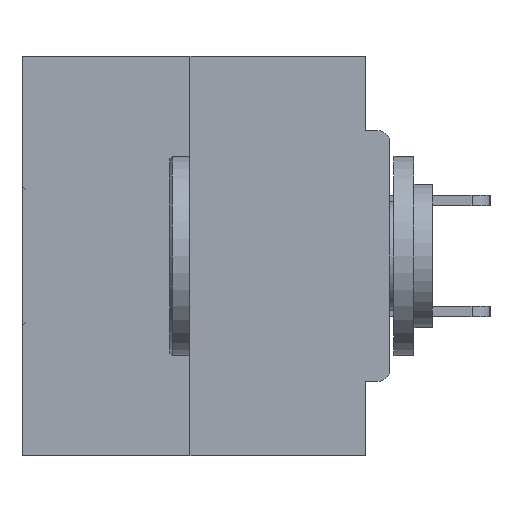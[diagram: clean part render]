
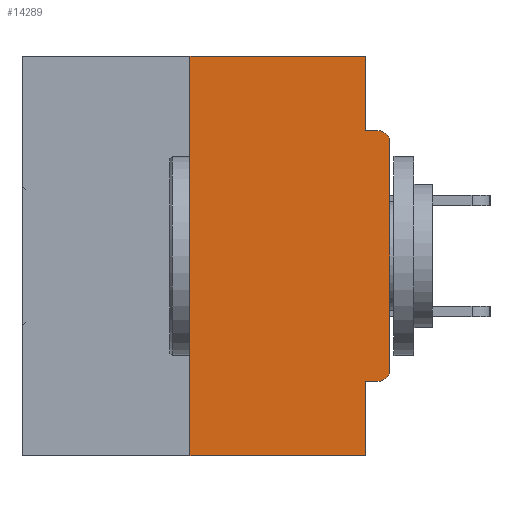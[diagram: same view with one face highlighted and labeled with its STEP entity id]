
A CAD part, left-side view. The second image highlights one B-rep face of the part: STEP entity #14289.
In plain terms, the highlighted planar face has unit normal (-1, 0, 0).
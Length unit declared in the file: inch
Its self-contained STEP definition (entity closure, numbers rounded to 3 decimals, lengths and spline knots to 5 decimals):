
#1080 = EDGE_CURVE ( 'NONE', #7391, #29625, #39101, .T. ) ;
#1329 = ORIENTED_EDGE ( 'NONE', *, *, #24493, .F. ) ;
#1868 = PLANE ( 'NONE',  #25152 ) ;
#2980 = VERTEX_POINT ( 'NONE', #11362 ) ;
#3025 = CARTESIAN_POINT ( 'NONE',  ( 0., 0.031, -0.5 ) ) ;
#3159 = CARTESIAN_POINT ( 'NONE',  ( 0., 0.015, -0.3915 ) ) ;
#3633 = EDGE_CURVE ( 'NONE', #15242, #29625, #30633, .T. ) ;
#3781 = EDGE_LOOP ( 'NONE', ( #1329, #34280, #20419, #6458, #30630, #20638, #4569, #37839, #4929, #18616 ) ) ;
#3794 = DIRECTION ( 'NONE',  ( 0., 0., -1. ) ) ;
#4330 = CARTESIAN_POINT ( 'NONE',  ( 0., 0., -0.1085 ) ) ;
#4569 = ORIENTED_EDGE ( 'NONE', *, *, #7837, .T. ) ;
#4770 = DIRECTION ( 'NONE',  ( 1., 0., 0. ) ) ;
#4929 = ORIENTED_EDGE ( 'NONE', *, *, #3633, .F. ) ;
#6458 = ORIENTED_EDGE ( 'NONE', *, *, #23088, .F. ) ;
#7391 = VERTEX_POINT ( 'NONE', #4330 ) ;
#7837 = EDGE_CURVE ( 'NONE', #17919, #7391, #25244, .T. ) ;
#8629 = LINE ( 'NONE', #20270, #10664 ) ;
#10664 = VECTOR ( 'NONE', #23188, 39.37008 ) ;
#10782 = CIRCLE ( 'NONE', #37553, 0.015 ) ;
#10955 = LINE ( 'NONE', #12834, #26357 ) ;
#11361 = DIRECTION ( 'NONE',  ( 0., 0., -1. ) ) ;
#11362 = CARTESIAN_POINT ( 'NONE',  ( 0., 0.015, -0.4065 ) ) ;
#11868 = VECTOR ( 'NONE', #3794, 39.37008 ) ;
#12834 = CARTESIAN_POINT ( 'NONE',  ( 0., 0., -0.4065 ) ) ;
#13036 = DIRECTION ( 'NONE',  ( -1., 0., 0. ) ) ;
#13815 = DIRECTION ( 'NONE',  ( 0., 0., 1. ) ) ;
#13870 = VERTEX_POINT ( 'NONE', #34517 ) ;
#14289 = ADVANCED_FACE ( 'NONE', ( #29590 ), #1868, .F. ) ;
#14334 = VECTOR ( 'NONE', #17943, 39.37008 ) ;
#14474 = CARTESIAN_POINT ( 'NONE',  ( 0., 0.46, -0.5 ) ) ;
#15218 = VECTOR ( 'NONE', #21391, 39.37008 ) ;
#15242 = VERTEX_POINT ( 'NONE', #38464 ) ;
#15964 = VECTOR ( 'NONE', #13815, 39.37008 ) ;
#16025 = CARTESIAN_POINT ( 'NONE',  ( 0., 0.015, -0.1085 ) ) ;
#17919 = VERTEX_POINT ( 'NONE', #25286 ) ;
#17943 = DIRECTION ( 'NONE',  ( 0., -1., 0. ) ) ;
#18616 = ORIENTED_EDGE ( 'NONE', *, *, #32157, .F. ) ;
#18814 = LINE ( 'NONE', #22248, #31158 ) ;
#19020 = LINE ( 'NONE', #23449, #11868 ) ;
#20270 = CARTESIAN_POINT ( 'NONE',  ( 0., 0.46, 0. ) ) ;
#20419 = ORIENTED_EDGE ( 'NONE', *, *, #38435, .T. ) ;
#20638 = ORIENTED_EDGE ( 'NONE', *, *, #38048, .T. ) ;
#21044 = LINE ( 'NONE', #14474, #14334 ) ;
#21241 = VERTEX_POINT ( 'NONE', #35505 ) ;
#21391 = DIRECTION ( 'NONE',  ( 0., -1., 0. ) ) ;
#22248 = CARTESIAN_POINT ( 'NONE',  ( 0., 0.25, 0. ) ) ;
#23088 = EDGE_CURVE ( 'NONE', #26156, #38046, #19020, .T. ) ;
#23188 = DIRECTION ( 'NONE',  ( 0., -1., 0. ) ) ;
#23449 = CARTESIAN_POINT ( 'NONE',  ( 0., 0.031, -0.5 ) ) ;
#23458 = CARTESIAN_POINT ( 'NONE',  ( 0., 0., 0. ) ) ;
#24069 = CARTESIAN_POINT ( 'NONE',  ( 0., 0.015, -0.0935 ) ) ;
#24268 = CARTESIAN_POINT ( 'NONE',  ( 0., 0., -0.0935 ) ) ;
#24421 = CARTESIAN_POINT ( 'NONE',  ( 0., 0.46, 0. ) ) ;
#24439 = LINE ( 'NONE', #29338, #42397 ) ;
#24493 = EDGE_CURVE ( 'NONE', #21241, #13870, #8629, .T. ) ;
#25152 = AXIS2_PLACEMENT_3D ( 'NONE', #24421, #4770, #11361 ) ;
#25244 = LINE ( 'NONE', #23458, #15964 ) ;
#25286 = CARTESIAN_POINT ( 'NONE',  ( 0., 0., -0.3915 ) ) ;
#25393 = DIRECTION ( 'NONE',  ( 0., 0., 1. ) ) ;
#25832 = DIRECTION ( 'NONE',  ( 0., 0., -1. ) ) ;
#26156 = VERTEX_POINT ( 'NONE', #39070 ) ;
#26357 = VECTOR ( 'NONE', #35253, 39.37008 ) ;
#28271 = VERTEX_POINT ( 'NONE', #33080 ) ;
#29338 = CARTESIAN_POINT ( 'NONE',  ( 0., 0.031, 0. ) ) ;
#29430 = DIRECTION ( 'NONE',  ( 0., 0., -1. ) ) ;
#29590 = FACE_OUTER_BOUND ( 'NONE', #3781, .T. ) ;
#29625 = VERTEX_POINT ( 'NONE', #24069 ) ;
#30630 = ORIENTED_EDGE ( 'NONE', *, *, #33194, .F. ) ;
#30633 = LINE ( 'NONE', #24268, #15218 ) ;
#31158 = VECTOR ( 'NONE', #25393, 39.37008 ) ;
#31517 = EDGE_CURVE ( 'NONE', #28271, #21241, #18814, .T. ) ;
#32157 = EDGE_CURVE ( 'NONE', #13870, #15242, #24439, .T. ) ;
#33080 = CARTESIAN_POINT ( 'NONE',  ( 0., 0.25, -0.5 ) ) ;
#33194 = EDGE_CURVE ( 'NONE', #2980, #26156, #10955, .T. ) ;
#33919 = AXIS2_PLACEMENT_3D ( 'NONE', #16025, #13036, #25832 ) ;
#34280 = ORIENTED_EDGE ( 'NONE', *, *, #31517, .F. ) ;
#34517 = CARTESIAN_POINT ( 'NONE',  ( 0., 0.031, 0. ) ) ;
#35253 = DIRECTION ( 'NONE',  ( 0., 1., 0. ) ) ;
#35505 = CARTESIAN_POINT ( 'NONE',  ( 0., 0.25, 0. ) ) ;
#37553 = AXIS2_PLACEMENT_3D ( 'NONE', #3159, #39312, #29430 ) ;
#37839 = ORIENTED_EDGE ( 'NONE', *, *, #1080, .T. ) ;
#38046 = VERTEX_POINT ( 'NONE', #3025 ) ;
#38048 = EDGE_CURVE ( 'NONE', #2980, #17919, #10782, .T. ) ;
#38435 = EDGE_CURVE ( 'NONE', #28271, #38046, #21044, .T. ) ;
#38464 = CARTESIAN_POINT ( 'NONE',  ( 0., 0.031, -0.0935 ) ) ;
#39070 = CARTESIAN_POINT ( 'NONE',  ( 0., 0.031, -0.4065 ) ) ;
#39101 = CIRCLE ( 'NONE', #33919, 0.015 ) ;
#39312 = DIRECTION ( 'NONE',  ( -1., 0., 0. ) ) ;
#39356 = DIRECTION ( 'NONE',  ( 0., 0., -1. ) ) ;
#42397 = VECTOR ( 'NONE', #39356, 39.37008 ) ;
